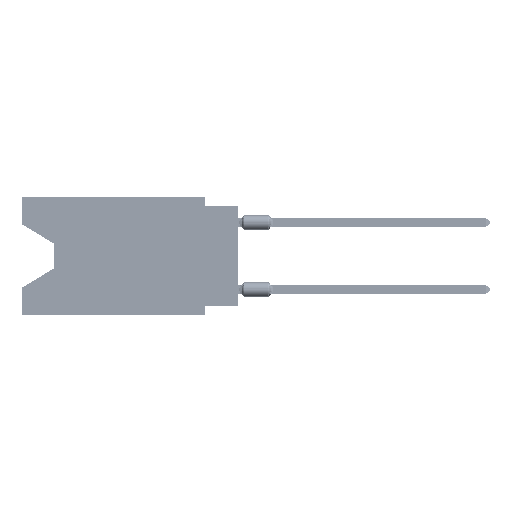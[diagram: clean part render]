
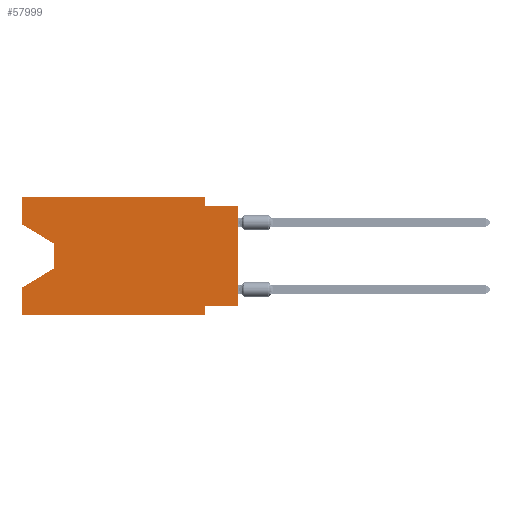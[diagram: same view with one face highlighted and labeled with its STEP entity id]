
A CAD part, left-side view. The second image highlights one B-rep face of the part: STEP entity #57999.
In plain terms, the highlighted planar face has unit normal (-1, 0, 0).
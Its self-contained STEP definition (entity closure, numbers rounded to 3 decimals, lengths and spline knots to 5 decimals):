
#460 = VECTOR ( 'NONE', #20228, 39.37008 ) ;
#782 = EDGE_CURVE ( 'NONE', #12935, #14961, #70260, .T. ) ;
#3838 = CARTESIAN_POINT ( 'NONE',  ( 0., 0.1, 0. ) ) ;
#4363 = EDGE_CURVE ( 'NONE', #91403, #102980, #87335, .T. ) ;
#5083 = FACE_OUTER_BOUND ( 'NONE', #64695, .T. ) ;
#8035 = DIRECTION ( 'NONE',  ( 0., -1., 0. ) ) ;
#8201 = VECTOR ( 'NONE', #8035, 39.37008 ) ;
#9864 = CARTESIAN_POINT ( 'NONE',  ( 0., 0.645, -0.08025 ) ) ;
#10889 = CARTESIAN_POINT ( 'NONE',  ( 0., 0.55, -0.138 ) ) ;
#12105 = LINE ( 'NONE', #17874, #8201 ) ;
#12873 = CARTESIAN_POINT ( 'NONE',  ( 0., 0.645, 0. ) ) ;
#12935 = VERTEX_POINT ( 'NONE', #116491 ) ;
#14961 = VERTEX_POINT ( 'NONE', #103957 ) ;
#16660 = VERTEX_POINT ( 'NONE', #24969 ) ;
#17149 = CARTESIAN_POINT ( 'NONE',  ( 0., 0.1, -0.35 ) ) ;
#17874 = CARTESIAN_POINT ( 'NONE',  ( 0., 0.645, 0. ) ) ;
#17918 = DIRECTION ( 'NONE',  ( 0., 0., 1. ) ) ;
#20228 = DIRECTION ( 'NONE',  ( 0., 1., 0. ) ) ;
#20737 = DIRECTION ( 'NONE',  ( 0., 0., -1. ) ) ;
#21002 = VERTEX_POINT ( 'NONE', #74786 ) ;
#24078 = ORIENTED_EDGE ( 'NONE', *, *, #26400, .T. ) ;
#24969 = CARTESIAN_POINT ( 'NONE',  ( 0., 0.1, 0. ) ) ;
#25730 = CARTESIAN_POINT ( 'NONE',  ( 0., 0.645, -0.08025 ) ) ;
#26231 = EDGE_CURVE ( 'NONE', #21002, #27730, #119652, .T. ) ;
#26394 = LINE ( 'NONE', #17149, #101903 ) ;
#26400 = EDGE_CURVE ( 'NONE', #89538, #78402, #83292, .T. ) ;
#26553 = ORIENTED_EDGE ( 'NONE', *, *, #26231, .F. ) ;
#27730 = VERTEX_POINT ( 'NONE', #36545 ) ;
#28342 = EDGE_CURVE ( 'NONE', #91403, #27730, #120805, .T. ) ;
#31943 = ORIENTED_EDGE ( 'NONE', *, *, #76697, .F. ) ;
#31975 = ORIENTED_EDGE ( 'NONE', *, *, #67545, .F. ) ;
#32320 = EDGE_CURVE ( 'NONE', #80621, #50448, #46490, .T. ) ;
#36393 = CARTESIAN_POINT ( 'NONE',  ( 0., 0., 0. ) ) ;
#36545 = CARTESIAN_POINT ( 'NONE',  ( 0., 0., -0.025 ) ) ;
#37744 = LINE ( 'NONE', #12873, #70357 ) ;
#38339 = DIRECTION ( 'NONE',  ( 0., 0., 1. ) ) ;
#38696 = CARTESIAN_POINT ( 'NONE',  ( 0., 0., -0.325 ) ) ;
#40215 = CARTESIAN_POINT ( 'NONE',  ( 0., 0.645, 0. ) ) ;
#41414 = DIRECTION ( 'NONE',  ( 0., 0., -1. ) ) ;
#43849 = EDGE_CURVE ( 'NONE', #16660, #21002, #50659, .T. ) ;
#44902 = ORIENTED_EDGE ( 'NONE', *, *, #91579, .T. ) ;
#45428 = LINE ( 'NONE', #25730, #93037 ) ;
#46490 = LINE ( 'NONE', #84074, #60088 ) ;
#49110 = ORIENTED_EDGE ( 'NONE', *, *, #117885, .T. ) ;
#50448 = VERTEX_POINT ( 'NONE', #56602 ) ;
#50496 = VECTOR ( 'NONE', #41414, 39.37008 ) ;
#50659 = LINE ( 'NONE', #3838, #50496 ) ;
#54095 = ORIENTED_EDGE ( 'NONE', *, *, #4363, .F. ) ;
#54343 = CARTESIAN_POINT ( 'NONE',  ( 0., 0.55, -0.212 ) ) ;
#56602 = CARTESIAN_POINT ( 'NONE',  ( 0., 0.645, 0. ) ) ;
#57999 = ADVANCED_FACE ( 'NONE', ( #5083 ), #59324, .F. ) ;
#59324 = PLANE ( 'NONE',  #99593 ) ;
#60088 = VECTOR ( 'NONE', #121650, 39.37008 ) ;
#60757 = VECTOR ( 'NONE', #17918, 39.37008 ) ;
#61366 = VECTOR ( 'NONE', #89345, 39.37008 ) ;
#62160 = CARTESIAN_POINT ( 'NONE',  ( 0., 0.55, -0.138 ) ) ;
#62231 = CARTESIAN_POINT ( 'NONE',  ( 0., 0.645, -0.35 ) ) ;
#64695 = EDGE_LOOP ( 'NONE', ( #49110, #44902, #24078, #102940, #65539, #31943, #54095, #70668, #26553, #117049, #31975, #75433 ) ) ;
#65539 = ORIENTED_EDGE ( 'NONE', *, *, #782, .T. ) ;
#67545 = EDGE_CURVE ( 'NONE', #50448, #16660, #12105, .T. ) ;
#70260 = LINE ( 'NONE', #62231, #61366 ) ;
#70357 = VECTOR ( 'NONE', #38339, 39.37008 ) ;
#70404 = DIRECTION ( 'NONE',  ( 0., 0., -1. ) ) ;
#70668 = ORIENTED_EDGE ( 'NONE', *, *, #28342, .T. ) ;
#74786 = CARTESIAN_POINT ( 'NONE',  ( 0., 0.1, -0.025 ) ) ;
#75433 = ORIENTED_EDGE ( 'NONE', *, *, #32320, .F. ) ;
#76697 = EDGE_CURVE ( 'NONE', #102980, #14961, #26394, .T. ) ;
#77799 = DIRECTION ( 'NONE',  ( 1., 0., 0. ) ) ;
#78402 = VERTEX_POINT ( 'NONE', #82508 ) ;
#80611 = CARTESIAN_POINT ( 'NONE',  ( 0., 0., -0.325 ) ) ;
#80621 = VERTEX_POINT ( 'NONE', #9864 ) ;
#82508 = CARTESIAN_POINT ( 'NONE',  ( 0., 0.645, -0.26975 ) ) ;
#83292 = LINE ( 'NONE', #54343, #113785 ) ;
#84074 = CARTESIAN_POINT ( 'NONE',  ( 0., 0.645, 0. ) ) ;
#84497 = EDGE_CURVE ( 'NONE', #12935, #78402, #37744, .T. ) ;
#87335 = LINE ( 'NONE', #38696, #460 ) ;
#89345 = DIRECTION ( 'NONE',  ( 0., -1., 0. ) ) ;
#89538 = VERTEX_POINT ( 'NONE', #96364 ) ;
#91403 = VERTEX_POINT ( 'NONE', #80611 ) ;
#91579 = EDGE_CURVE ( 'NONE', #119874, #89538, #111968, .T. ) ;
#93037 = VECTOR ( 'NONE', #121176, 39.37008 ) ;
#94000 = VECTOR ( 'NONE', #20737, 39.37008 ) ;
#96364 = CARTESIAN_POINT ( 'NONE',  ( 0., 0.55, -0.212 ) ) ;
#98123 = CARTESIAN_POINT ( 'NONE',  ( 0., 0., -0.025 ) ) ;
#99593 = AXIS2_PLACEMENT_3D ( 'NONE', #40215, #77799, #70404 ) ;
#99963 = DIRECTION ( 'NONE',  ( 0., -1., 0. ) ) ;
#99989 = VECTOR ( 'NONE', #99963, 39.37008 ) ;
#101903 = VECTOR ( 'NONE', #121251, 39.37008 ) ;
#102940 = ORIENTED_EDGE ( 'NONE', *, *, #84497, .F. ) ;
#102975 = DIRECTION ( 'NONE',  ( 0., 0.855, -0.519 ) ) ;
#102980 = VERTEX_POINT ( 'NONE', #119753 ) ;
#103957 = CARTESIAN_POINT ( 'NONE',  ( 0., 0.1, -0.35 ) ) ;
#111968 = LINE ( 'NONE', #10889, #94000 ) ;
#113785 = VECTOR ( 'NONE', #102975, 39.37008 ) ;
#116491 = CARTESIAN_POINT ( 'NONE',  ( 0., 0.645, -0.35 ) ) ;
#117049 = ORIENTED_EDGE ( 'NONE', *, *, #43849, .F. ) ;
#117885 = EDGE_CURVE ( 'NONE', #80621, #119874, #45428, .T. ) ;
#119652 = LINE ( 'NONE', #98123, #99989 ) ;
#119753 = CARTESIAN_POINT ( 'NONE',  ( 0., 0.1, -0.325 ) ) ;
#119874 = VERTEX_POINT ( 'NONE', #62160 ) ;
#120805 = LINE ( 'NONE', #36393, #60757 ) ;
#121176 = DIRECTION ( 'NONE',  ( 0., -0.855, -0.519 ) ) ;
#121251 = DIRECTION ( 'NONE',  ( 0., 0., -1. ) ) ;
#121650 = DIRECTION ( 'NONE',  ( 0., 0., 1. ) ) ;
